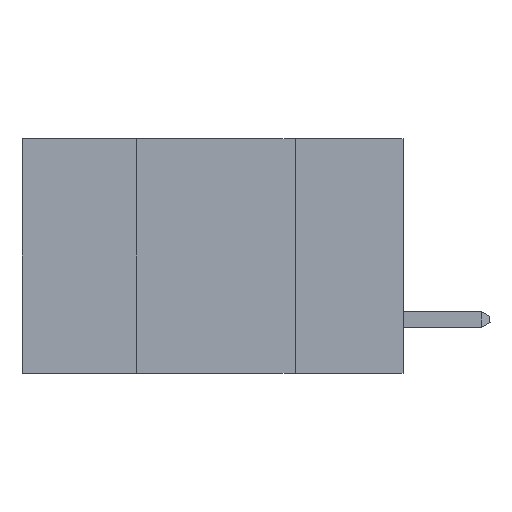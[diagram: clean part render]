
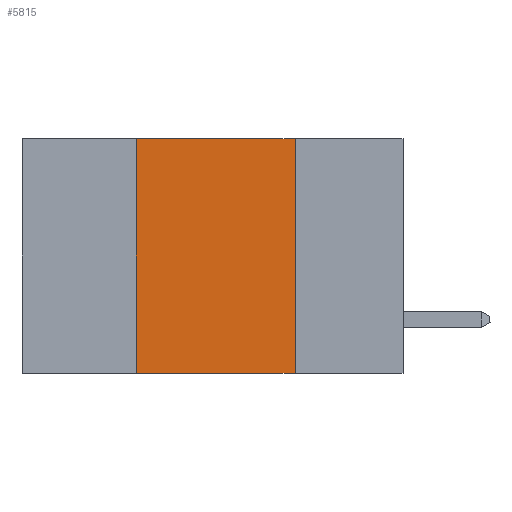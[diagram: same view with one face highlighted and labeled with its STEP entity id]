
A CAD part, left-side view. The second image highlights one B-rep face of the part: STEP entity #5815.
In plain terms, the highlighted planar face has unit normal (-1, 0, 0).
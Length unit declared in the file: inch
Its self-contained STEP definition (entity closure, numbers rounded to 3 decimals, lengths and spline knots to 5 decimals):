
#398 = AXIS2_PLACEMENT_3D ( 'NONE', #5354, #7764, #3074 ) ;
#566 = VERTEX_POINT ( 'NONE', #6881 ) ;
#582 = CARTESIAN_POINT ( 'NONE',  ( 0., 0.42, 0. ) ) ;
#701 = PLANE ( 'NONE',  #398 ) ;
#742 = ORIENTED_EDGE ( 'NONE', *, *, #7531, .F. ) ;
#1705 = VECTOR ( 'NONE', #1910, 39.37008 ) ;
#1910 = DIRECTION ( 'NONE',  ( 0., 0., -1. ) ) ;
#2053 = CARTESIAN_POINT ( 'NONE',  ( 0., 0.17, 0. ) ) ;
#2183 = DIRECTION ( 'NONE',  ( 0., 0., 1. ) ) ;
#2236 = CARTESIAN_POINT ( 'NONE',  ( 0., 0.42, 0. ) ) ;
#2456 = VECTOR ( 'NONE', #5531, 39.37008 ) ;
#2766 = EDGE_CURVE ( 'NONE', #8819, #6751, #7273, .T. ) ;
#3074 = DIRECTION ( 'NONE',  ( 0., 0., -1. ) ) ;
#3298 = CARTESIAN_POINT ( 'NONE',  ( 0., 0.6, -0.37 ) ) ;
#3403 = ORIENTED_EDGE ( 'NONE', *, *, #7519, .T. ) ;
#3753 = CARTESIAN_POINT ( 'NONE',  ( 0., 0.17, -0.37 ) ) ;
#4770 = LINE ( 'NONE', #7233, #2456 ) ;
#5236 = LINE ( 'NONE', #2053, #1705 ) ;
#5354 = CARTESIAN_POINT ( 'NONE',  ( 0., 0.6, 0. ) ) ;
#5531 = DIRECTION ( 'NONE',  ( 0., -1., 0. ) ) ;
#5716 = EDGE_LOOP ( 'NONE', ( #7156, #742, #7365, #3403 ) ) ;
#5815 = ADVANCED_FACE ( 'NONE', ( #8715 ), #701, .F. ) ;
#6067 = VECTOR ( 'NONE', #2183, 39.37008 ) ;
#6239 = VECTOR ( 'NONE', #9538, 39.37008 ) ;
#6751 = VERTEX_POINT ( 'NONE', #582 ) ;
#6881 = CARTESIAN_POINT ( 'NONE',  ( 0., 0.17, 0. ) ) ;
#6971 = LINE ( 'NONE', #3298, #6239 ) ;
#7156 = ORIENTED_EDGE ( 'NONE', *, *, #8441, .F. ) ;
#7233 = CARTESIAN_POINT ( 'NONE',  ( 0., 0.6, 0. ) ) ;
#7273 = LINE ( 'NONE', #2236, #6067 ) ;
#7365 = ORIENTED_EDGE ( 'NONE', *, *, #2766, .F. ) ;
#7519 = EDGE_CURVE ( 'NONE', #8819, #7999, #6971, .T. ) ;
#7531 = EDGE_CURVE ( 'NONE', #6751, #566, #4770, .T. ) ;
#7764 = DIRECTION ( 'NONE',  ( 1., 0., 0. ) ) ;
#7999 = VERTEX_POINT ( 'NONE', #3753 ) ;
#8441 = EDGE_CURVE ( 'NONE', #566, #7999, #5236, .T. ) ;
#8715 = FACE_OUTER_BOUND ( 'NONE', #5716, .T. ) ;
#8819 = VERTEX_POINT ( 'NONE', #9734 ) ;
#9538 = DIRECTION ( 'NONE',  ( 0., -1., 0. ) ) ;
#9734 = CARTESIAN_POINT ( 'NONE',  ( 0., 0.42, -0.37 ) ) ;
